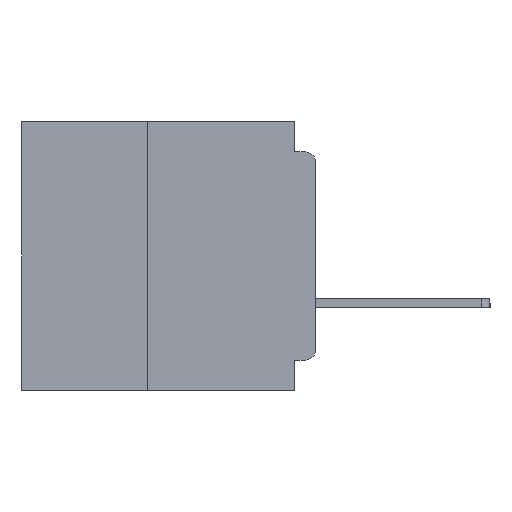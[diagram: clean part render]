
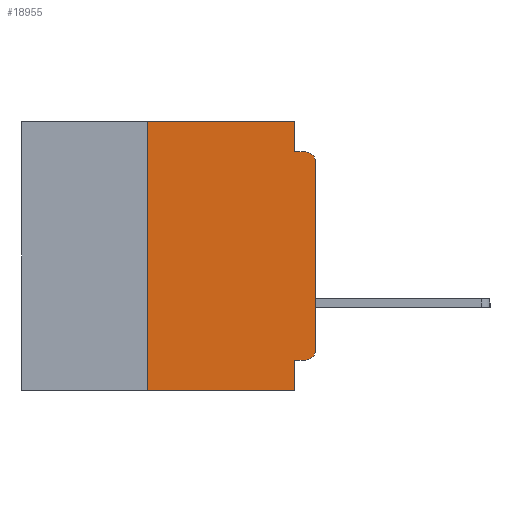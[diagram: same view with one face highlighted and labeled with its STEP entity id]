
A CAD part, left-side view. The second image highlights one B-rep face of the part: STEP entity #18955.
In plain terms, the highlighted planar face has unit normal (-1, 0, 0).
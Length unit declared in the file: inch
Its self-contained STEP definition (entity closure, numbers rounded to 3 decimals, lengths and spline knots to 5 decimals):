
#5 = VERTEX_POINT ( 'NONE', #28268 ) ;
#166 = CARTESIAN_POINT ( 'NONE',  ( 0., 0., -0.045 ) ) ;
#491 = CARTESIAN_POINT ( 'NONE',  ( 0., 0.25, -0.4 ) ) ;
#517 = CARTESIAN_POINT ( 'NONE',  ( 0., 0.015, -0.06 ) ) ;
#1265 = ORIENTED_EDGE ( 'NONE', *, *, #1839, .F. ) ;
#1700 = CARTESIAN_POINT ( 'NONE',  ( 0., 0.25, 0. ) ) ;
#1728 = DIRECTION ( 'NONE',  ( -1., 0., 0. ) ) ;
#1839 = EDGE_CURVE ( 'NONE', #25290, #24089, #23892, .T. ) ;
#2301 = VECTOR ( 'NONE', #12443, 39.37008 ) ;
#2688 = CARTESIAN_POINT ( 'NONE',  ( 0., 0.015, -0.045 ) ) ;
#2820 = DIRECTION ( 'NONE',  ( 1., 0., 0. ) ) ;
#3366 = DIRECTION ( 'NONE',  ( 0., -1., 0. ) ) ;
#3562 = CARTESIAN_POINT ( 'NONE',  ( 0., 0.031, -0.355 ) ) ;
#3726 = DIRECTION ( 'NONE',  ( 0., 0., -1. ) ) ;
#4880 = VECTOR ( 'NONE', #6069, 39.37008 ) ;
#5080 = VERTEX_POINT ( 'NONE', #24993 ) ;
#5411 = LINE ( 'NONE', #27059, #12934 ) ;
#6069 = DIRECTION ( 'NONE',  ( 0., 0., 1. ) ) ;
#6214 = CARTESIAN_POINT ( 'NONE',  ( 0., 0.031, 0. ) ) ;
#8718 = CARTESIAN_POINT ( 'NONE',  ( 0., 0., 0. ) ) ;
#9017 = AXIS2_PLACEMENT_3D ( 'NONE', #20879, #1728, #24064 ) ;
#9899 = EDGE_CURVE ( 'NONE', #36378, #5080, #5411, .T. ) ;
#10204 = EDGE_CURVE ( 'NONE', #24104, #17274, #37019, .T. ) ;
#10785 = LINE ( 'NONE', #12304, #2301 ) ;
#11303 = EDGE_CURVE ( 'NONE', #24104, #5, #10785, .T. ) ;
#12129 = ORIENTED_EDGE ( 'NONE', *, *, #30665, .F. ) ;
#12196 = CARTESIAN_POINT ( 'NONE',  ( 0., 0.437, 0. ) ) ;
#12304 = CARTESIAN_POINT ( 'NONE',  ( 0., 0.437, -0.4 ) ) ;
#12443 = DIRECTION ( 'NONE',  ( 0., -1., 0. ) ) ;
#12934 = VECTOR ( 'NONE', #36842, 39.37008 ) ;
#13043 = CIRCLE ( 'NONE', #9017, 0.015 ) ;
#16040 = CIRCLE ( 'NONE', #22948, 0.015 ) ;
#16275 = LINE ( 'NONE', #166, #32350 ) ;
#17274 = VERTEX_POINT ( 'NONE', #1700 ) ;
#17464 = DIRECTION ( 'NONE',  ( 0., 0., -1. ) ) ;
#17872 = VECTOR ( 'NONE', #17464, 39.37008 ) ;
#18884 = ORIENTED_EDGE ( 'NONE', *, *, #40323, .T. ) ;
#18945 = VERTEX_POINT ( 'NONE', #2688 ) ;
#18955 = ADVANCED_FACE ( 'NONE', ( #31349 ), #34788, .F. ) ;
#19369 = LINE ( 'NONE', #28450, #26837 ) ;
#20686 = CARTESIAN_POINT ( 'NONE',  ( 0., 0.031, -0.4 ) ) ;
#20879 = CARTESIAN_POINT ( 'NONE',  ( 0., 0.015, -0.34 ) ) ;
#22009 = CARTESIAN_POINT ( 'NONE',  ( 0., 0.25, -0.4 ) ) ;
#22887 = DIRECTION ( 'NONE',  ( -1., 0., 0. ) ) ;
#22948 = AXIS2_PLACEMENT_3D ( 'NONE', #517, #22887, #3726 ) ;
#23062 = CARTESIAN_POINT ( 'NONE',  ( 0., 0., -0.355 ) ) ;
#23892 = LINE ( 'NONE', #23062, #24876 ) ;
#24064 = DIRECTION ( 'NONE',  ( 0., 0., -1. ) ) ;
#24089 = VERTEX_POINT ( 'NONE', #3562 ) ;
#24104 = VERTEX_POINT ( 'NONE', #491 ) ;
#24876 = VECTOR ( 'NONE', #28195, 39.37008 ) ;
#24993 = CARTESIAN_POINT ( 'NONE',  ( 0., 0.031, -0.045 ) ) ;
#25153 = DIRECTION ( 'NONE',  ( 0., 0., -1. ) ) ;
#25290 = VERTEX_POINT ( 'NONE', #33707 ) ;
#26634 = ORIENTED_EDGE ( 'NONE', *, *, #11303, .T. ) ;
#26837 = VECTOR ( 'NONE', #38061, 39.37008 ) ;
#27059 = CARTESIAN_POINT ( 'NONE',  ( 0., 0.031, 0. ) ) ;
#27328 = CARTESIAN_POINT ( 'NONE',  ( 0., 0., -0.34 ) ) ;
#28195 = DIRECTION ( 'NONE',  ( 0., 1., 0. ) ) ;
#28268 = CARTESIAN_POINT ( 'NONE',  ( 0., 0.031, -0.4 ) ) ;
#28281 = ORIENTED_EDGE ( 'NONE', *, *, #9899, .F. ) ;
#28450 = CARTESIAN_POINT ( 'NONE',  ( 0., 0.437, 0. ) ) ;
#30422 = EDGE_LOOP ( 'NONE', ( #36534, #18884, #40101, #28281, #31337, #40437, #26634, #12129, #1265, #31051 ) ) ;
#30665 = EDGE_CURVE ( 'NONE', #24089, #5, #34966, .T. ) ;
#31051 = ORIENTED_EDGE ( 'NONE', *, *, #31855, .T. ) ;
#31168 = DIRECTION ( 'NONE',  ( 0., 0., 1. ) ) ;
#31337 = ORIENTED_EDGE ( 'NONE', *, *, #33657, .F. ) ;
#31349 = FACE_OUTER_BOUND ( 'NONE', #30422, .T. ) ;
#31855 = EDGE_CURVE ( 'NONE', #25290, #36170, #13043, .T. ) ;
#31965 = VECTOR ( 'NONE', #31168, 39.37008 ) ;
#32350 = VECTOR ( 'NONE', #3366, 39.37008 ) ;
#33537 = EDGE_CURVE ( 'NONE', #36170, #36185, #40467, .T. ) ;
#33657 = EDGE_CURVE ( 'NONE', #17274, #36378, #19369, .T. ) ;
#33707 = CARTESIAN_POINT ( 'NONE',  ( 0., 0.015, -0.355 ) ) ;
#33735 = CARTESIAN_POINT ( 'NONE',  ( 0., 0., -0.06 ) ) ;
#34788 = PLANE ( 'NONE',  #35089 ) ;
#34966 = LINE ( 'NONE', #20686, #17872 ) ;
#35089 = AXIS2_PLACEMENT_3D ( 'NONE', #12196, #2820, #25153 ) ;
#36170 = VERTEX_POINT ( 'NONE', #27328 ) ;
#36185 = VERTEX_POINT ( 'NONE', #33735 ) ;
#36378 = VERTEX_POINT ( 'NONE', #6214 ) ;
#36534 = ORIENTED_EDGE ( 'NONE', *, *, #33537, .T. ) ;
#36842 = DIRECTION ( 'NONE',  ( 0., 0., -1. ) ) ;
#37019 = LINE ( 'NONE', #22009, #4880 ) ;
#37094 = EDGE_CURVE ( 'NONE', #5080, #18945, #16275, .T. ) ;
#38061 = DIRECTION ( 'NONE',  ( 0., -1., 0. ) ) ;
#40101 = ORIENTED_EDGE ( 'NONE', *, *, #37094, .F. ) ;
#40323 = EDGE_CURVE ( 'NONE', #36185, #18945, #16040, .T. ) ;
#40437 = ORIENTED_EDGE ( 'NONE', *, *, #10204, .F. ) ;
#40467 = LINE ( 'NONE', #8718, #31965 ) ;
